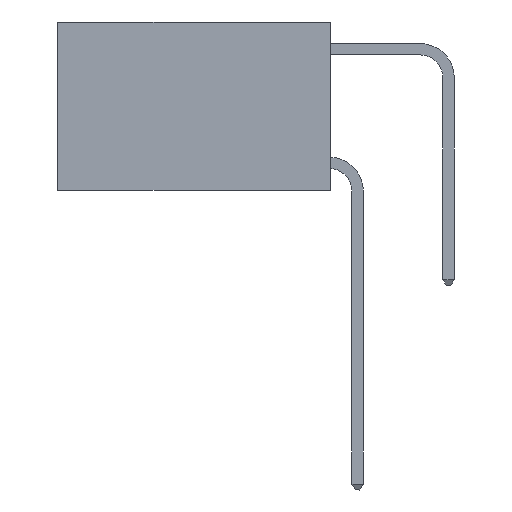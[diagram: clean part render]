
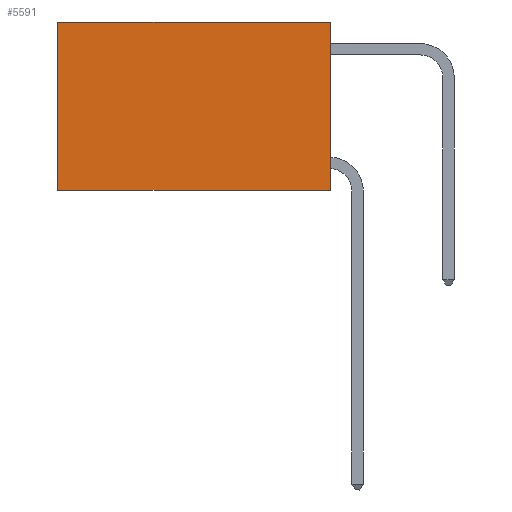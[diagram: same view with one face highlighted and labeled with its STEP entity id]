
A CAD part, left-side view. The second image highlights one B-rep face of the part: STEP entity #5591.
In plain terms, the highlighted planar face has unit normal (-1, 0, 0).
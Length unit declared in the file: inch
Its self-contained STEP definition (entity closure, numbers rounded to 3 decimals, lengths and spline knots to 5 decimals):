
#134 = ORIENTED_EDGE ( 'NONE', *, *, #11268, .F. ) ;
#345 = LINE ( 'NONE', #7238, #8056 ) ;
#1070 = CARTESIAN_POINT ( 'NONE',  ( 0.2625, 0., -0.37 ) ) ;
#1085 = CARTESIAN_POINT ( 'NONE',  ( 0.2625, 0., 0. ) ) ;
#1703 = LINE ( 'NONE', #3961, #12623 ) ;
#1832 = DIRECTION ( 'NONE',  ( 1., 0., 0. ) ) ;
#2384 = LINE ( 'NONE', #8075, #9356 ) ;
#3961 = CARTESIAN_POINT ( 'NONE',  ( 0.2625, 0., 0. ) ) ;
#3988 = ORIENTED_EDGE ( 'NONE', *, *, #10453, .T. ) ;
#4874 = DIRECTION ( 'NONE',  ( 0., 0., -1. ) ) ;
#5138 = ORIENTED_EDGE ( 'NONE', *, *, #8312, .F. ) ;
#5284 = ORIENTED_EDGE ( 'NONE', *, *, #9796, .T. ) ;
#5591 = ADVANCED_FACE ( 'NONE', ( #6811 ), #7959, .F. ) ;
#6219 = DIRECTION ( 'NONE',  ( 0., 0., -1. ) ) ;
#6271 = DIRECTION ( 'NONE',  ( 0., 1., 0. ) ) ;
#6449 = VERTEX_POINT ( 'NONE', #1070 ) ;
#6811 = FACE_OUTER_BOUND ( 'NONE', #7846, .T. ) ;
#7238 = CARTESIAN_POINT ( 'NONE',  ( 0.2625, 0., -0.37 ) ) ;
#7558 = CARTESIAN_POINT ( 'NONE',  ( 0.2625, 0.6, 0. ) ) ;
#7846 = EDGE_LOOP ( 'NONE', ( #3988, #134, #5138, #5284 ) ) ;
#7959 = PLANE ( 'NONE',  #11875 ) ;
#8056 = VECTOR ( 'NONE', #9582, 39.37008 ) ;
#8075 = CARTESIAN_POINT ( 'NONE',  ( 0.2625, 0., 0. ) ) ;
#8312 = EDGE_CURVE ( 'NONE', #10656, #6449, #2384, .T. ) ;
#8996 = VECTOR ( 'NONE', #6219, 39.37008 ) ;
#9356 = VECTOR ( 'NONE', #4874, 39.37008 ) ;
#9582 = DIRECTION ( 'NONE',  ( 0., 1., 0. ) ) ;
#9796 = EDGE_CURVE ( 'NONE', #10656, #11394, #1703, .T. ) ;
#10453 = EDGE_CURVE ( 'NONE', #11394, #14156, #14246, .T. ) ;
#10645 = CARTESIAN_POINT ( 'NONE',  ( 0.2625, 0.6, 0. ) ) ;
#10656 = VERTEX_POINT ( 'NONE', #1085 ) ;
#11268 = EDGE_CURVE ( 'NONE', #6449, #14156, #345, .T. ) ;
#11394 = VERTEX_POINT ( 'NONE', #10645 ) ;
#11523 = DIRECTION ( 'NONE',  ( 0., 0., -1. ) ) ;
#11875 = AXIS2_PLACEMENT_3D ( 'NONE', #14855, #1832, #11523 ) ;
#12175 = CARTESIAN_POINT ( 'NONE',  ( 0.2625, 0.6, -0.37 ) ) ;
#12623 = VECTOR ( 'NONE', #6271, 39.37008 ) ;
#14156 = VERTEX_POINT ( 'NONE', #12175 ) ;
#14246 = LINE ( 'NONE', #7558, #8996 ) ;
#14855 = CARTESIAN_POINT ( 'NONE',  ( 0.2625, 0., 0. ) ) ;
